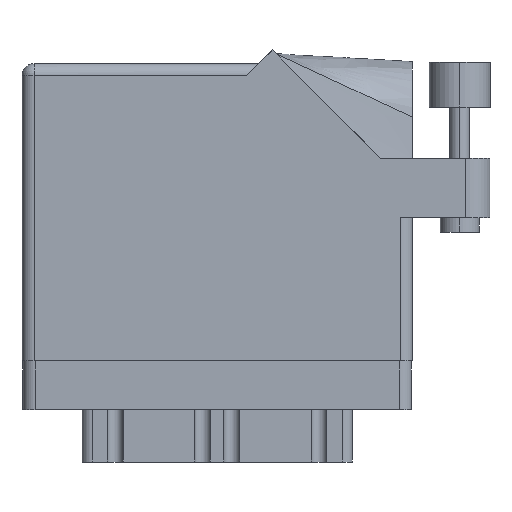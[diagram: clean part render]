
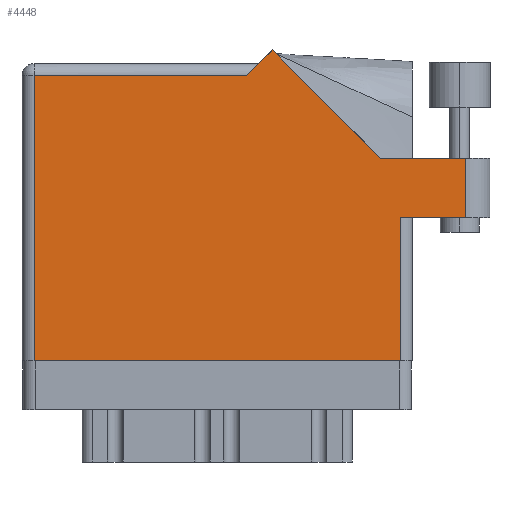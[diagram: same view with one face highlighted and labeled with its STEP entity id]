
A CAD part, front view. The second image highlights one B-rep face of the part: STEP entity #4448.
In plain terms, the highlighted face is planar.
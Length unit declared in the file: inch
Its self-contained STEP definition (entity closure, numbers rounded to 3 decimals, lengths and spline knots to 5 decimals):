
#78 = EDGE_CURVE ( 'NONE', #27406, #14074, #2690, .T. ) ;
#449 = DIRECTION ( 'NONE',  ( -1., 0., 0. ) ) ;
#1161 = CARTESIAN_POINT ( 'NONE',  ( 0., 0., 0. ) ) ;
#2129 = CARTESIAN_POINT ( 'NONE',  ( 1.948, 0., 0. ) ) ;
#2298 = CARTESIAN_POINT ( 'NONE',  ( 1.217, 1.53, 0. ) ) ;
#2690 = LINE ( 'NONE', #24248, #13564 ) ;
#3101 = CARTESIAN_POINT ( 'NONE',  ( 2.285, 1.044, 0. ) ) ;
#3285 = LINE ( 'NONE', #15458, #9669 ) ;
#3658 = ORIENTED_EDGE ( 'NONE', *, *, #6449, .T. ) ;
#3891 = CARTESIAN_POINT ( 'NONE',  ( 0.062, 1.468, 0. ) ) ;
#3964 = ORIENTED_EDGE ( 'NONE', *, *, #78, .T. ) ;
#4448 = ADVANCED_FACE ( 'NONE', ( #22125 ), #6017, .F. ) ;
#4476 = CARTESIAN_POINT ( 'NONE',  ( 2.285, 0.737, 0. ) ) ;
#4670 = CARTESIAN_POINT ( 'NONE',  ( 2.41, 1.044, 0. ) ) ;
#4972 = LINE ( 'NONE', #4670, #18184 ) ;
#5230 = DIRECTION ( 'NONE',  ( 0., 1., 0. ) ) ;
#5447 = LINE ( 'NONE', #14665, #30102 ) ;
#6017 = PLANE ( 'NONE',  #20998 ) ;
#6140 = VERTEX_POINT ( 'NONE', #7759 ) ;
#6150 = CARTESIAN_POINT ( 'NONE',  ( 1.84442, 1.044, 0. ) ) ;
#6449 = EDGE_CURVE ( 'NONE', #22028, #6140, #26621, .T. ) ;
#7283 = LINE ( 'NONE', #16827, #18553 ) ;
#7759 = CARTESIAN_POINT ( 'NONE',  ( 1.948, 0.737, 0. ) ) ;
#8475 = CARTESIAN_POINT ( 'NONE',  ( 1.28771, 1.60071, 0. ) ) ;
#9161 = VERTEX_POINT ( 'NONE', #13863 ) ;
#9552 = ORIENTED_EDGE ( 'NONE', *, *, #19318, .T. ) ;
#9669 = VECTOR ( 'NONE', #29969, 39.37008 ) ;
#10374 = CARTESIAN_POINT ( 'NONE',  ( 1.948, 0.737, 0. ) ) ;
#11414 = ORIENTED_EDGE ( 'NONE', *, *, #19829, .T. ) ;
#12024 = VECTOR ( 'NONE', #12324, 39.37008 ) ;
#12320 = DIRECTION ( 'NONE',  ( -0.707, 0.707, 0. ) ) ;
#12324 = DIRECTION ( 'NONE',  ( 0., -1., 0. ) ) ;
#12369 = DIRECTION ( 'NONE',  ( 0., 1., 0. ) ) ;
#12717 = EDGE_CURVE ( 'NONE', #26339, #16198, #5447, .T. ) ;
#12902 = CARTESIAN_POINT ( 'NONE',  ( 0., 1.53, 0. ) ) ;
#13174 = LINE ( 'NONE', #1161, #28815 ) ;
#13564 = VECTOR ( 'NONE', #12369, 39.37008 ) ;
#13863 = CARTESIAN_POINT ( 'NONE',  ( 0.062, 0., 0. ) ) ;
#14074 = VERTEX_POINT ( 'NONE', #3101 ) ;
#14215 = CARTESIAN_POINT ( 'NONE',  ( 0.062, 0., 0. ) ) ;
#14665 = CARTESIAN_POINT ( 'NONE',  ( 1.84442, 1.044, 0. ) ) ;
#15087 = DIRECTION ( 'NONE',  ( -1., 0., 0. ) ) ;
#15244 = DIRECTION ( 'NONE',  ( 0., 0., -1. ) ) ;
#15458 = CARTESIAN_POINT ( 'NONE',  ( 0., 1.468, 0. ) ) ;
#15848 = VERTEX_POINT ( 'NONE', #3891 ) ;
#15855 = ORIENTED_EDGE ( 'NONE', *, *, #16181, .T. ) ;
#16181 = EDGE_CURVE ( 'NONE', #9161, #22028, #13174, .T. ) ;
#16198 = VERTEX_POINT ( 'NONE', #8475 ) ;
#16827 = CARTESIAN_POINT ( 'NONE',  ( 2.01, 0.737, 0. ) ) ;
#17051 = ORIENTED_EDGE ( 'NONE', *, *, #22513, .T. ) ;
#18184 = VECTOR ( 'NONE', #449, 39.37008 ) ;
#18553 = VECTOR ( 'NONE', #26190, 39.37008 ) ;
#19158 = DIRECTION ( 'NONE',  ( -0.707, -0.707, 0. ) ) ;
#19318 = EDGE_CURVE ( 'NONE', #15848, #9161, #28573, .T. ) ;
#19829 = EDGE_CURVE ( 'NONE', #6140, #27406, #7283, .T. ) ;
#20998 = AXIS2_PLACEMENT_3D ( 'NONE', #12902, #15244, #15087 ) ;
#21817 = LINE ( 'NONE', #2298, #26088 ) ;
#22028 = VERTEX_POINT ( 'NONE', #2129 ) ;
#22125 = FACE_OUTER_BOUND ( 'NONE', #23535, .T. ) ;
#22221 = ORIENTED_EDGE ( 'NONE', *, *, #12717, .T. ) ;
#22513 = EDGE_CURVE ( 'NONE', #25113, #15848, #3285, .T. ) ;
#22709 = CARTESIAN_POINT ( 'NONE',  ( 1.155, 1.468, 0. ) ) ;
#22719 = DIRECTION ( 'NONE',  ( 1., 0., 0. ) ) ;
#22768 = VECTOR ( 'NONE', #5230, 39.37008 ) ;
#22806 = EDGE_CURVE ( 'NONE', #14074, #26339, #4972, .T. ) ;
#23255 = EDGE_CURVE ( 'NONE', #16198, #25113, #21817, .T. ) ;
#23535 = EDGE_LOOP ( 'NONE', ( #11414, #3964, #28575, #22221, #24818, #17051, #9552, #15855, #3658 ) ) ;
#24248 = CARTESIAN_POINT ( 'NONE',  ( 2.285, 1.044, 0. ) ) ;
#24818 = ORIENTED_EDGE ( 'NONE', *, *, #23255, .T. ) ;
#25113 = VERTEX_POINT ( 'NONE', #22709 ) ;
#26088 = VECTOR ( 'NONE', #19158, 39.37008 ) ;
#26190 = DIRECTION ( 'NONE',  ( 1., 0., 0. ) ) ;
#26339 = VERTEX_POINT ( 'NONE', #6150 ) ;
#26621 = LINE ( 'NONE', #10374, #22768 ) ;
#27406 = VERTEX_POINT ( 'NONE', #4476 ) ;
#28573 = LINE ( 'NONE', #14215, #12024 ) ;
#28575 = ORIENTED_EDGE ( 'NONE', *, *, #22806, .T. ) ;
#28815 = VECTOR ( 'NONE', #22719, 39.37008 ) ;
#29969 = DIRECTION ( 'NONE',  ( -1., 0., 0. ) ) ;
#30102 = VECTOR ( 'NONE', #12320, 39.37008 ) ;
